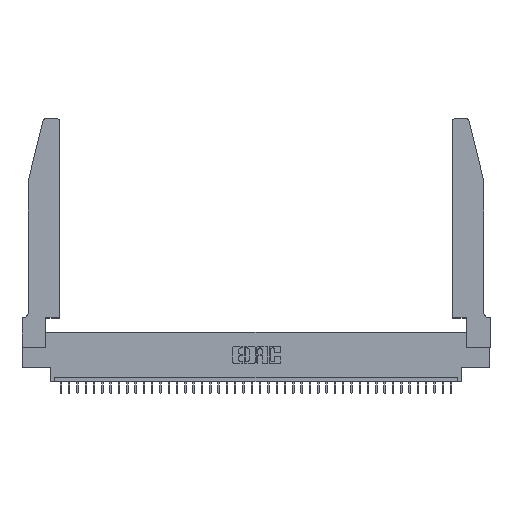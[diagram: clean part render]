
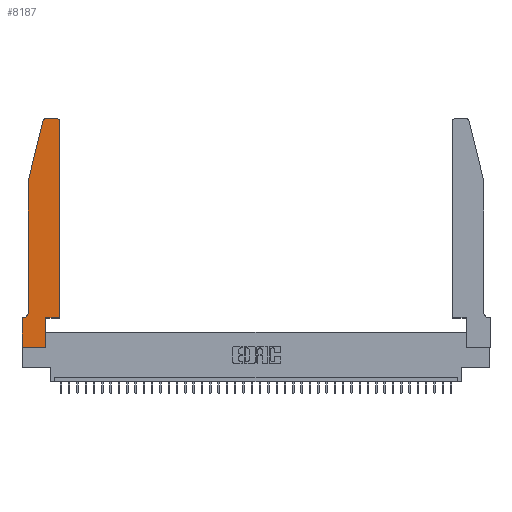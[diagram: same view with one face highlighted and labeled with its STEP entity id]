
A CAD part, top view. The second image highlights one B-rep face of the part: STEP entity #8187.
In plain terms, the highlighted planar face has unit normal (0, 0, 1).
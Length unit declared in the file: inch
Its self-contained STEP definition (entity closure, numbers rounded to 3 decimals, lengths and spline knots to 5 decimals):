
#209 = CARTESIAN_POINT ( 'NONE',  ( 0., 0., 0.37 ) ) ;
#217 = VECTOR ( 'NONE', #7306, 39.37008 ) ;
#680 = VECTOR ( 'NONE', #8810, 39.37008 ) ;
#928 = CARTESIAN_POINT ( 'NONE',  ( 0.4505, 2.72, 0.37 ) ) ;
#1470 = VERTEX_POINT ( 'NONE', #22928 ) ;
#1891 = FACE_OUTER_BOUND ( 'NONE', #24721, .T. ) ;
#2180 = DIRECTION ( 'NONE',  ( -1., 0., 0. ) ) ;
#2516 = LINE ( 'NONE', #14996, #16175 ) ;
#3651 = ORIENTED_EDGE ( 'NONE', *, *, #26105, .T. ) ;
#4180 = VERTEX_POINT ( 'NONE', #11322 ) ;
#4467 = EDGE_CURVE ( 'NONE', #16324, #23793, #31227, .T. ) ;
#5498 = DIRECTION ( 'NONE',  ( 1., 0., 0. ) ) ;
#5543 = LINE ( 'NONE', #30477, #680 ) ;
#6103 = CARTESIAN_POINT ( 'NONE',  ( 0.284, 2.72, 0.37 ) ) ;
#6192 = LINE ( 'NONE', #15793, #13990 ) ;
#6710 = EDGE_CURVE ( 'NONE', #28617, #35479, #7647, .T. ) ;
#7246 = ORIENTED_EDGE ( 'NONE', *, *, #11335, .T. ) ;
#7306 = DIRECTION ( 'NONE',  ( 1., 0., 0. ) ) ;
#7647 = LINE ( 'NONE', #20125, #24733 ) ;
#7753 = EDGE_CURVE ( 'NONE', #35479, #15384, #5543, .T. ) ;
#7836 = CARTESIAN_POINT ( 'NONE',  ( 0.2865, 0., 0.37 ) ) ;
#8187 = ADVANCED_FACE ( 'NONE', ( #1891 ), #39612, .T. ) ;
#8390 = AXIS2_PLACEMENT_3D ( 'NONE', #17220, #13941, #39418 ) ;
#8489 = EDGE_CURVE ( 'NONE', #37698, #28749, #22293, .T. ) ;
#8810 = DIRECTION ( 'NONE',  ( 0., 1., 0. ) ) ;
#9335 = VECTOR ( 'NONE', #15530, 39.37008 ) ;
#10156 = CARTESIAN_POINT ( 'NONE',  ( 0.2865, 0.35, 0.37 ) ) ;
#11322 = CARTESIAN_POINT ( 'NONE',  ( 0.0055, 0.35, 0.37 ) ) ;
#11335 = EDGE_CURVE ( 'NONE', #16676, #28617, #16703, .T. ) ;
#11528 = EDGE_CURVE ( 'NONE', #35831, #4180, #37934, .T. ) ;
#11762 = VECTOR ( 'NONE', #19417, 39.37008 ) ;
#11981 = CARTESIAN_POINT ( 'NONE',  ( 0., 0., 0.37 ) ) ;
#12627 = EDGE_CURVE ( 'NONE', #23793, #16676, #34673, .T. ) ;
#13334 = ORIENTED_EDGE ( 'NONE', *, *, #31087, .T. ) ;
#13588 = CIRCLE ( 'NONE', #8390, 0.03 ) ;
#13941 = DIRECTION ( 'NONE',  ( 0., 0., 1. ) ) ;
#13990 = VECTOR ( 'NONE', #22334, 39.37008 ) ;
#14375 = EDGE_CURVE ( 'NONE', #34005, #1470, #6192, .T. ) ;
#14996 = CARTESIAN_POINT ( 'NONE',  ( 0.0755, 2., 0.37 ) ) ;
#15330 = CARTESIAN_POINT ( 'NONE',  ( 0.0755, 0.35, 0.37 ) ) ;
#15384 = VERTEX_POINT ( 'NONE', #928 ) ;
#15530 = DIRECTION ( 'NONE',  ( -1., 0., 0. ) ) ;
#15793 = CARTESIAN_POINT ( 'NONE',  ( 0.0755, 2., 0.37 ) ) ;
#15914 = ORIENTED_EDGE ( 'NONE', *, *, #4467, .T. ) ;
#16175 = VECTOR ( 'NONE', #27474, 39.37008 ) ;
#16291 = CIRCLE ( 'NONE', #24099, 0.03 ) ;
#16324 = VERTEX_POINT ( 'NONE', #26547 ) ;
#16676 = VERTEX_POINT ( 'NONE', #7836 ) ;
#16703 = LINE ( 'NONE', #10156, #36632 ) ;
#16709 = CARTESIAN_POINT ( 'NONE',  ( 0.4505, 0.35, 0.37 ) ) ;
#16905 = DIRECTION ( 'NONE',  ( 0., 0., -1. ) ) ;
#17220 = CARTESIAN_POINT ( 'NONE',  ( 0.4205, 2.72, 0.37 ) ) ;
#17253 = ORIENTED_EDGE ( 'NONE', *, *, #32407, .T. ) ;
#17438 = ORIENTED_EDGE ( 'NONE', *, *, #6710, .T. ) ;
#18377 = DIRECTION ( 'NONE',  ( 0., -1., 0. ) ) ;
#19417 = DIRECTION ( 'NONE',  ( -1., 0., 0. ) ) ;
#19524 = CARTESIAN_POINT ( 'NONE',  ( 0.0755, 0.42, 0.37 ) ) ;
#19559 = DIRECTION ( 'NONE',  ( 0., 1., 0. ) ) ;
#19590 = ORIENTED_EDGE ( 'NONE', *, *, #14375, .T. ) ;
#20125 = CARTESIAN_POINT ( 'NONE',  ( 0.4505, 0.35, 0.37 ) ) ;
#20350 = AXIS2_PLACEMENT_3D ( 'NONE', #29954, #16905, #2180 ) ;
#21070 = CARTESIAN_POINT ( 'NONE',  ( 0., 0.35, 0.37 ) ) ;
#21334 = VECTOR ( 'NONE', #18377, 39.37008 ) ;
#21346 = ORIENTED_EDGE ( 'NONE', *, *, #12627, .T. ) ;
#21627 = DIRECTION ( 'NONE',  ( 0., 0., 1. ) ) ;
#22293 = LINE ( 'NONE', #34725, #11762 ) ;
#22334 = DIRECTION ( 'NONE',  ( -0.239, -0.971, 0. ) ) ;
#22928 = CARTESIAN_POINT ( 'NONE',  ( 0.0755, 2., 0.37 ) ) ;
#23793 = VERTEX_POINT ( 'NONE', #11981 ) ;
#24058 = CARTESIAN_POINT ( 'NONE',  ( 0.284, 2.75, 0.37 ) ) ;
#24099 = AXIS2_PLACEMENT_3D ( 'NONE', #6103, #21627, #5498 ) ;
#24145 = DIRECTION ( 'NONE',  ( 0., 0., 1. ) ) ;
#24721 = EDGE_LOOP ( 'NONE', ( #33623, #26347, #19590, #13334, #29195, #3651, #15914, #21346, #7246, #17438, #27713, #17253 ) ) ;
#24733 = VECTOR ( 'NONE', #38479, 39.37008 ) ;
#25915 = CARTESIAN_POINT ( 'NONE',  ( 0., 0., 0.37 ) ) ;
#26105 = EDGE_CURVE ( 'NONE', #4180, #16324, #36942, .T. ) ;
#26347 = ORIENTED_EDGE ( 'NONE', *, *, #33087, .T. ) ;
#26547 = CARTESIAN_POINT ( 'NONE',  ( 0., 0.35, 0.37 ) ) ;
#27474 = DIRECTION ( 'NONE',  ( 0., -1., 0. ) ) ;
#27713 = ORIENTED_EDGE ( 'NONE', *, *, #7753, .T. ) ;
#28491 = CARTESIAN_POINT ( 'NONE',  ( 0.25487, 2.72718, 0.37 ) ) ;
#28617 = VERTEX_POINT ( 'NONE', #35485 ) ;
#28749 = VERTEX_POINT ( 'NONE', #24058 ) ;
#29195 = ORIENTED_EDGE ( 'NONE', *, *, #11528, .T. ) ;
#29389 = AXIS2_PLACEMENT_3D ( 'NONE', #21070, #24145, #33121 ) ;
#29954 = CARTESIAN_POINT ( 'NONE',  ( 0.0055, 0.42, 0.37 ) ) ;
#30477 = CARTESIAN_POINT ( 'NONE',  ( 0.4505, 0.35, 0.37 ) ) ;
#31087 = EDGE_CURVE ( 'NONE', #1470, #35831, #2516, .T. ) ;
#31227 = LINE ( 'NONE', #209, #21334 ) ;
#32407 = EDGE_CURVE ( 'NONE', #15384, #37698, #13588, .T. ) ;
#33087 = EDGE_CURVE ( 'NONE', #28749, #34005, #16291, .T. ) ;
#33121 = DIRECTION ( 'NONE',  ( 1., 0., 0. ) ) ;
#33623 = ORIENTED_EDGE ( 'NONE', *, *, #8489, .T. ) ;
#34005 = VERTEX_POINT ( 'NONE', #28491 ) ;
#34673 = LINE ( 'NONE', #25915, #217 ) ;
#34725 = CARTESIAN_POINT ( 'NONE',  ( 0.2605, 2.75, 0.37 ) ) ;
#35479 = VERTEX_POINT ( 'NONE', #16709 ) ;
#35485 = CARTESIAN_POINT ( 'NONE',  ( 0.2865, 0.35, 0.37 ) ) ;
#35579 = CARTESIAN_POINT ( 'NONE',  ( 0.4205, 2.75, 0.37 ) ) ;
#35831 = VERTEX_POINT ( 'NONE', #19524 ) ;
#36632 = VECTOR ( 'NONE', #19559, 39.37008 ) ;
#36942 = LINE ( 'NONE', #15330, #9335 ) ;
#37698 = VERTEX_POINT ( 'NONE', #35579 ) ;
#37934 = CIRCLE ( 'NONE', #20350, 0.07 ) ;
#38479 = DIRECTION ( 'NONE',  ( 1., 0., 0. ) ) ;
#39418 = DIRECTION ( 'NONE',  ( 1., 0., 0. ) ) ;
#39612 = PLANE ( 'NONE',  #29389 ) ;
